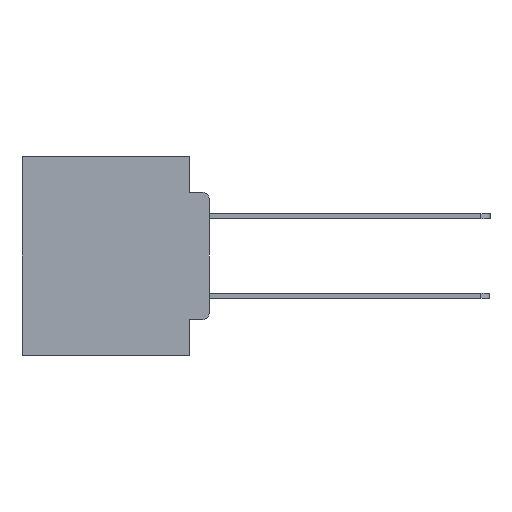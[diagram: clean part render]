
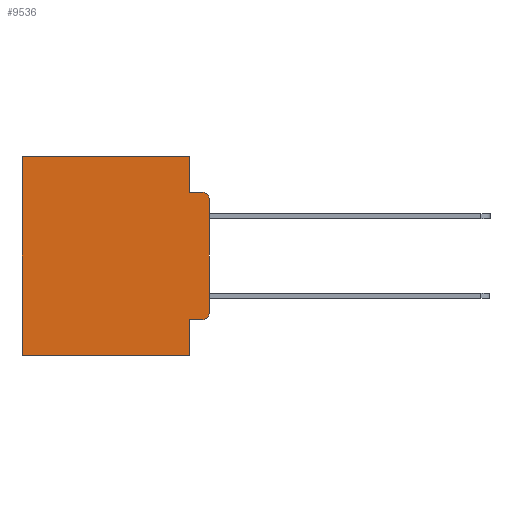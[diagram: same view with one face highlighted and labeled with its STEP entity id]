
A CAD part, left-side view. The second image highlights one B-rep face of the part: STEP entity #9536.
In plain terms, the highlighted planar face has unit normal (-1, 0, 0).
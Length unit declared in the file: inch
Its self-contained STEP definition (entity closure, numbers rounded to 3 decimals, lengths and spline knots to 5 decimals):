
#4 = LINE ( 'NONE', #5679, #12057 ) ;
#260 = CARTESIAN_POINT ( 'NONE',  ( 0.298, 0.051, 0. ) ) ;
#494 = CARTESIAN_POINT ( 'NONE',  ( 0.298, 0.02, -0.0885 ) ) ;
#576 = VERTEX_POINT ( 'NONE', #494 ) ;
#790 = ORIENTED_EDGE ( 'NONE', *, *, #20620, .T. ) ;
#1066 = LINE ( 'NONE', #18489, #6841 ) ;
#1895 = VERTEX_POINT ( 'NONE', #7182 ) ;
#2022 = VERTEX_POINT ( 'NONE', #17381 ) ;
#2544 = EDGE_CURVE ( 'NONE', #9154, #30428, #4, .T. ) ;
#2742 = DIRECTION ( 'NONE',  ( 0., 0., -1. ) ) ;
#2901 = VECTOR ( 'NONE', #30296, 39.37008 ) ;
#3026 = LINE ( 'NONE', #260, #14955 ) ;
#4050 = VECTOR ( 'NONE', #9861, 39.37008 ) ;
#4357 = CARTESIAN_POINT ( 'NONE',  ( 0.298, 0.051, 0. ) ) ;
#4952 = EDGE_CURVE ( 'NONE', #30428, #2022, #28954, .T. ) ;
#5474 = EDGE_LOOP ( 'NONE', ( #12445, #11509, #11446, #23120, #21289, #19628, #19133, #18368, #18317, #790 ) ) ;
#5679 = CARTESIAN_POINT ( 'NONE',  ( 0.298, 0., 0. ) ) ;
#5854 = PLANE ( 'NONE',  #23048 ) ;
#6815 = DIRECTION ( 'NONE',  ( 0., -1., 0. ) ) ;
#6841 = VECTOR ( 'NONE', #6815, 39.37008 ) ;
#7182 = CARTESIAN_POINT ( 'NONE',  ( 0.298, 0., -0.1085 ) ) ;
#7293 = CARTESIAN_POINT ( 'NONE',  ( 0.298, 0.051, -0.5 ) ) ;
#7384 = EDGE_CURVE ( 'NONE', #27141, #11893, #16201, .T. ) ;
#7439 = CARTESIAN_POINT ( 'NONE',  ( 0.298, 0.02, -0.4115 ) ) ;
#8271 = DIRECTION ( 'NONE',  ( 1., 0., 0. ) ) ;
#8899 = CARTESIAN_POINT ( 'NONE',  ( 0.298, 0.051, -0.0885 ) ) ;
#9154 = VERTEX_POINT ( 'NONE', #23208 ) ;
#9233 = DIRECTION ( 'NONE',  ( 0., 1., 0. ) ) ;
#9392 = CARTESIAN_POINT ( 'NONE',  ( 0.298, 0., -0.5 ) ) ;
#9536 = ADVANCED_FACE ( 'NONE', ( #17526 ), #5854, .F. ) ;
#9861 = DIRECTION ( 'NONE',  ( 0., 0., -1. ) ) ;
#10672 = VERTEX_POINT ( 'NONE', #7293 ) ;
#10729 = CARTESIAN_POINT ( 'NONE',  ( 0.298, 0., 0. ) ) ;
#10757 = CARTESIAN_POINT ( 'NONE',  ( 0.298, 0.051, -0.4115 ) ) ;
#11247 = EDGE_CURVE ( 'NONE', #10672, #2022, #22512, .T. ) ;
#11263 = DIRECTION ( 'NONE',  ( -1., 0., 0. ) ) ;
#11446 = ORIENTED_EDGE ( 'NONE', *, *, #15239, .F. ) ;
#11509 = ORIENTED_EDGE ( 'NONE', *, *, #23522, .T. ) ;
#11832 = CARTESIAN_POINT ( 'NONE',  ( 0.298, 0.473, 0. ) ) ;
#11893 = VERTEX_POINT ( 'NONE', #7439 ) ;
#12057 = VECTOR ( 'NONE', #9233, 39.37008 ) ;
#12166 = EDGE_CURVE ( 'NONE', #9154, #22883, #3026, .T. ) ;
#12445 = ORIENTED_EDGE ( 'NONE', *, *, #22146, .F. ) ;
#12829 = CARTESIAN_POINT ( 'NONE',  ( 0.298, 0., 0. ) ) ;
#13304 = CARTESIAN_POINT ( 'NONE',  ( 0.298, 0.02, -0.3915 ) ) ;
#13395 = VECTOR ( 'NONE', #24746, 39.37008 ) ;
#14955 = VECTOR ( 'NONE', #2742, 39.37008 ) ;
#15239 = EDGE_CURVE ( 'NONE', #22883, #576, #1066, .T. ) ;
#15706 = DIRECTION ( 'NONE',  ( 0., 0., -1. ) ) ;
#16201 = LINE ( 'NONE', #27811, #21707 ) ;
#17196 = CIRCLE ( 'NONE', #18047, 0.02 ) ;
#17381 = CARTESIAN_POINT ( 'NONE',  ( 0.298, 0.473, -0.5 ) ) ;
#17526 = FACE_OUTER_BOUND ( 'NONE', #5474, .T. ) ;
#17573 = VERTEX_POINT ( 'NONE', #28925 ) ;
#17815 = LINE ( 'NONE', #4357, #30089 ) ;
#18047 = AXIS2_PLACEMENT_3D ( 'NONE', #25260, #11263, #27581 ) ;
#18317 = ORIENTED_EDGE ( 'NONE', *, *, #7384, .T. ) ;
#18368 = ORIENTED_EDGE ( 'NONE', *, *, #25247, .F. ) ;
#18489 = CARTESIAN_POINT ( 'NONE',  ( 0.298, 0.051, -0.0885 ) ) ;
#18623 = DIRECTION ( 'NONE',  ( 0., -1., 0. ) ) ;
#18769 = AXIS2_PLACEMENT_3D ( 'NONE', #13304, #29552, #15706 ) ;
#19133 = ORIENTED_EDGE ( 'NONE', *, *, #11247, .F. ) ;
#19628 = ORIENTED_EDGE ( 'NONE', *, *, #4952, .T. ) ;
#20395 = LINE ( 'NONE', #10729, #13395 ) ;
#20620 = EDGE_CURVE ( 'NONE', #11893, #17573, #29463, .T. ) ;
#21289 = ORIENTED_EDGE ( 'NONE', *, *, #2544, .T. ) ;
#21707 = VECTOR ( 'NONE', #18623, 39.37008 ) ;
#22146 = EDGE_CURVE ( 'NONE', #1895, #17573, #20395, .T. ) ;
#22512 = LINE ( 'NONE', #9392, #2901 ) ;
#22883 = VERTEX_POINT ( 'NONE', #8899 ) ;
#23048 = AXIS2_PLACEMENT_3D ( 'NONE', #12829, #8271, #24580 ) ;
#23120 = ORIENTED_EDGE ( 'NONE', *, *, #12166, .F. ) ;
#23206 = DIRECTION ( 'NONE',  ( 0., 0., -1. ) ) ;
#23208 = CARTESIAN_POINT ( 'NONE',  ( 0.298, 0.051, 0. ) ) ;
#23522 = EDGE_CURVE ( 'NONE', #1895, #576, #17196, .T. ) ;
#23870 = CARTESIAN_POINT ( 'NONE',  ( 0.298, 0.473, 0. ) ) ;
#24580 = DIRECTION ( 'NONE',  ( 0., 0., -1. ) ) ;
#24746 = DIRECTION ( 'NONE',  ( 0., 0., -1. ) ) ;
#25247 = EDGE_CURVE ( 'NONE', #27141, #10672, #17815, .T. ) ;
#25260 = CARTESIAN_POINT ( 'NONE',  ( 0.298, 0.02, -0.1085 ) ) ;
#27141 = VERTEX_POINT ( 'NONE', #10757 ) ;
#27581 = DIRECTION ( 'NONE',  ( 0., 0., -1. ) ) ;
#27811 = CARTESIAN_POINT ( 'NONE',  ( 0.298, 0.051, -0.4115 ) ) ;
#28925 = CARTESIAN_POINT ( 'NONE',  ( 0.298, 0., -0.3915 ) ) ;
#28954 = LINE ( 'NONE', #23870, #4050 ) ;
#29463 = CIRCLE ( 'NONE', #18769, 0.02 ) ;
#29552 = DIRECTION ( 'NONE',  ( -1., 0., 0. ) ) ;
#30089 = VECTOR ( 'NONE', #23206, 39.37008 ) ;
#30296 = DIRECTION ( 'NONE',  ( 0., 1., 0. ) ) ;
#30428 = VERTEX_POINT ( 'NONE', #11832 ) ;
